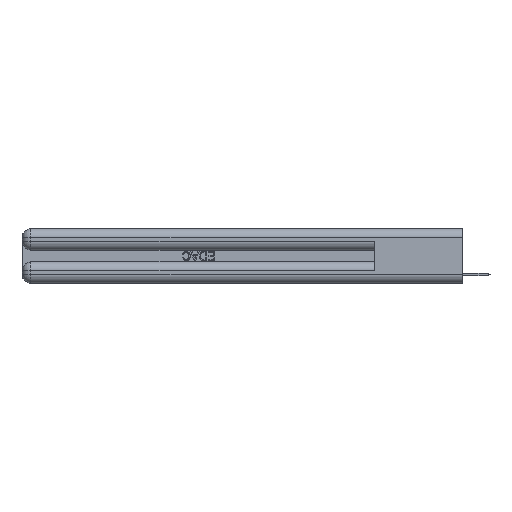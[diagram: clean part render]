
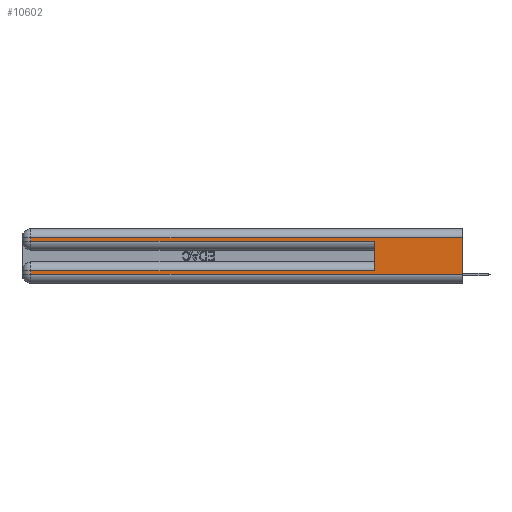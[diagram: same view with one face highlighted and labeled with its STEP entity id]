
A CAD part, left-side view. The second image highlights one B-rep face of the part: STEP entity #10602.
In plain terms, the highlighted planar face has unit normal (-1, 0, 0).
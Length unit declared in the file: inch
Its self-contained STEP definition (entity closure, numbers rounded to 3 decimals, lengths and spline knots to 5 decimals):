
#734 = LINE ( 'NONE', #22365, #14209 ) ;
#1414 = CARTESIAN_POINT ( 'NONE',  ( 0., 2.94, 0.06 ) ) ;
#1739 = LINE ( 'NONE', #31197, #12768 ) ;
#3079 = LINE ( 'NONE', #14170, #19383 ) ;
#3845 = VECTOR ( 'NONE', #5484, 39.37008 ) ;
#4628 = VERTEX_POINT ( 'NONE', #9119 ) ;
#5428 = EDGE_CURVE ( 'NONE', #27763, #5493, #734, .T. ) ;
#5484 = DIRECTION ( 'NONE',  ( 0., 0., -1. ) ) ;
#5493 = VERTEX_POINT ( 'NONE', #27065 ) ;
#5684 = DIRECTION ( 'NONE',  ( 0., 1., 0. ) ) ;
#6036 = VERTEX_POINT ( 'NONE', #26310 ) ;
#6435 = EDGE_CURVE ( 'NONE', #32374, #27763, #33691, .T. ) ;
#6591 = FACE_OUTER_BOUND ( 'NONE', #24520, .T. ) ;
#7588 = VECTOR ( 'NONE', #13266, 39.37008 ) ;
#7813 = ORIENTED_EDGE ( 'NONE', *, *, #19751, .F. ) ;
#8208 = CARTESIAN_POINT ( 'NONE',  ( 0., 2.94, 0.31 ) ) ;
#9119 = CARTESIAN_POINT ( 'NONE',  ( 0., 2.94, 0.085 ) ) ;
#9948 = CARTESIAN_POINT ( 'NONE',  ( 0., 2.94, 0.37 ) ) ;
#10490 = CARTESIAN_POINT ( 'NONE',  ( 0., 0., 0.06 ) ) ;
#10602 = ADVANCED_FACE ( 'NONE', ( #6591 ), #14582, .F. ) ;
#10854 = ORIENTED_EDGE ( 'NONE', *, *, #33434, .T. ) ;
#11340 = VERTEX_POINT ( 'NONE', #12075 ) ;
#12075 = CARTESIAN_POINT ( 'NONE',  ( 0., 0., 0.31 ) ) ;
#12157 = DIRECTION ( 'NONE',  ( 1., 0., 0. ) ) ;
#12768 = VECTOR ( 'NONE', #28945, 39.37008 ) ;
#13266 = DIRECTION ( 'NONE',  ( 0., -1., 0. ) ) ;
#13336 = VECTOR ( 'NONE', #33635, 39.37008 ) ;
#14170 = CARTESIAN_POINT ( 'NONE',  ( 0., 0., 0.085 ) ) ;
#14209 = VECTOR ( 'NONE', #21860, 39.37008 ) ;
#14367 = EDGE_CURVE ( 'NONE', #23848, #6036, #25906, .T. ) ;
#14582 = PLANE ( 'NONE',  #31446 ) ;
#15104 = CARTESIAN_POINT ( 'NONE',  ( 0., 0., 0.37 ) ) ;
#15450 = LINE ( 'NONE', #15104, #13336 ) ;
#15740 = CARTESIAN_POINT ( 'NONE',  ( 0., 2.94, 0.37 ) ) ;
#17405 = ORIENTED_EDGE ( 'NONE', *, *, #29264, .T. ) ;
#19132 = EDGE_CURVE ( 'NONE', #27402, #4628, #3079, .T. ) ;
#19383 = VECTOR ( 'NONE', #5684, 39.37008 ) ;
#19751 = EDGE_CURVE ( 'NONE', #27402, #5493, #1739, .T. ) ;
#20530 = DIRECTION ( 'NONE',  ( 0., 0., -1. ) ) ;
#21860 = DIRECTION ( 'NONE',  ( 0., -1., 0. ) ) ;
#22238 = LINE ( 'NONE', #32305, #31893 ) ;
#22365 = CARTESIAN_POINT ( 'NONE',  ( 0., 0., 0.285 ) ) ;
#22528 = DIRECTION ( 'NONE',  ( 0., 0., -1. ) ) ;
#22738 = CARTESIAN_POINT ( 'NONE',  ( 0., 0.6, 0.085 ) ) ;
#22876 = CARTESIAN_POINT ( 'NONE',  ( 0., 0., 0.37 ) ) ;
#23848 = VERTEX_POINT ( 'NONE', #1414 ) ;
#23954 = CARTESIAN_POINT ( 'NONE',  ( 0., 2.94, 0.285 ) ) ;
#24498 = DIRECTION ( 'NONE',  ( 0., 1., 0. ) ) ;
#24520 = EDGE_LOOP ( 'NONE', ( #28172, #17405, #25774, #34083, #7813, #32258, #10854, #32886 ) ) ;
#25774 = ORIENTED_EDGE ( 'NONE', *, *, #6435, .T. ) ;
#25906 = LINE ( 'NONE', #10490, #7588 ) ;
#26310 = CARTESIAN_POINT ( 'NONE',  ( 0., 0., 0.06 ) ) ;
#27065 = CARTESIAN_POINT ( 'NONE',  ( 0., 0.6, 0.285 ) ) ;
#27402 = VERTEX_POINT ( 'NONE', #22738 ) ;
#27511 = VECTOR ( 'NONE', #20530, 39.37008 ) ;
#27763 = VERTEX_POINT ( 'NONE', #23954 ) ;
#28172 = ORIENTED_EDGE ( 'NONE', *, *, #34060, .F. ) ;
#28945 = DIRECTION ( 'NONE',  ( 0., 0., 1. ) ) ;
#29066 = LINE ( 'NONE', #15740, #3845 ) ;
#29264 = EDGE_CURVE ( 'NONE', #11340, #32374, #22238, .T. ) ;
#31197 = CARTESIAN_POINT ( 'NONE',  ( 0., 0.6, 0.145 ) ) ;
#31446 = AXIS2_PLACEMENT_3D ( 'NONE', #22876, #12157, #22528 ) ;
#31893 = VECTOR ( 'NONE', #24498, 39.37008 ) ;
#32258 = ORIENTED_EDGE ( 'NONE', *, *, #19132, .T. ) ;
#32305 = CARTESIAN_POINT ( 'NONE',  ( 0., 0., 0.31 ) ) ;
#32374 = VERTEX_POINT ( 'NONE', #8208 ) ;
#32886 = ORIENTED_EDGE ( 'NONE', *, *, #14367, .T. ) ;
#33434 = EDGE_CURVE ( 'NONE', #4628, #23848, #29066, .T. ) ;
#33635 = DIRECTION ( 'NONE',  ( 0., 0., -1. ) ) ;
#33691 = LINE ( 'NONE', #9948, #27511 ) ;
#34060 = EDGE_CURVE ( 'NONE', #11340, #6036, #15450, .T. ) ;
#34083 = ORIENTED_EDGE ( 'NONE', *, *, #5428, .T. ) ;
